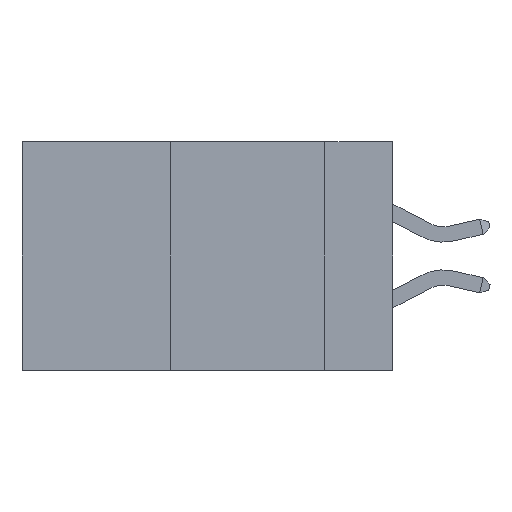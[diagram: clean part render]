
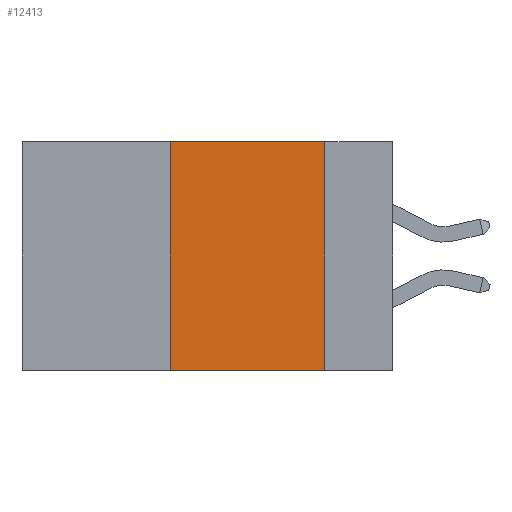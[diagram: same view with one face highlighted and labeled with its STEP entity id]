
A CAD part, left-side view. The second image highlights one B-rep face of the part: STEP entity #12413.
In plain terms, the highlighted planar face has unit normal (-1, 0, 0).
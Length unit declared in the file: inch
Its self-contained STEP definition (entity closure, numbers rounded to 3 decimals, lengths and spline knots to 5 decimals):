
#387 = LINE ( 'NONE', #16037, #11804 ) ;
#531 = EDGE_CURVE ( 'NONE', #13870, #1696, #387, .T. ) ;
#978 = CARTESIAN_POINT ( 'NONE',  ( 0., 0.6, -0.37 ) ) ;
#1008 = CARTESIAN_POINT ( 'NONE',  ( 0., 0.6, 0. ) ) ;
#1041 = EDGE_CURVE ( 'NONE', #1696, #4029, #7498, .T. ) ;
#1696 = VERTEX_POINT ( 'NONE', #3296 ) ;
#2862 = AXIS2_PLACEMENT_3D ( 'NONE', #1008, #8720, #8781 ) ;
#2865 = ORIENTED_EDGE ( 'NONE', *, *, #4188, .T. ) ;
#3212 = VERTEX_POINT ( 'NONE', #8947 ) ;
#3296 = CARTESIAN_POINT ( 'NONE',  ( 0., 0.11, 0. ) ) ;
#4016 = DIRECTION ( 'NONE',  ( 0., -1., 0. ) ) ;
#4029 = VERTEX_POINT ( 'NONE', #18912 ) ;
#4188 = EDGE_CURVE ( 'NONE', #3212, #4029, #18372, .T. ) ;
#6347 = CARTESIAN_POINT ( 'NONE',  ( 0., 0.11, 0. ) ) ;
#6585 = LINE ( 'NONE', #16337, #11335 ) ;
#7106 = FACE_OUTER_BOUND ( 'NONE', #11029, .T. ) ;
#7338 = ORIENTED_EDGE ( 'NONE', *, *, #531, .F. ) ;
#7498 = LINE ( 'NONE', #6347, #13186 ) ;
#8720 = DIRECTION ( 'NONE',  ( 1., 0., 0. ) ) ;
#8781 = DIRECTION ( 'NONE',  ( 0., 0., -1. ) ) ;
#8947 = CARTESIAN_POINT ( 'NONE',  ( 0., 0.36, -0.37 ) ) ;
#9289 = ORIENTED_EDGE ( 'NONE', *, *, #13616, .F. ) ;
#10104 = PLANE ( 'NONE',  #2862 ) ;
#10910 = DIRECTION ( 'NONE',  ( 0., 0., -1. ) ) ;
#11029 = EDGE_LOOP ( 'NONE', ( #13820, #7338, #9289, #2865 ) ) ;
#11335 = VECTOR ( 'NONE', #17888, 39.37008 ) ;
#11804 = VECTOR ( 'NONE', #19195, 39.37008 ) ;
#12413 = ADVANCED_FACE ( 'NONE', ( #7106 ), #10104, .F. ) ;
#13186 = VECTOR ( 'NONE', #10910, 39.37008 ) ;
#13616 = EDGE_CURVE ( 'NONE', #3212, #13870, #6585, .T. ) ;
#13820 = ORIENTED_EDGE ( 'NONE', *, *, #1041, .F. ) ;
#13870 = VERTEX_POINT ( 'NONE', #18229 ) ;
#16037 = CARTESIAN_POINT ( 'NONE',  ( 0., 0.6, 0. ) ) ;
#16337 = CARTESIAN_POINT ( 'NONE',  ( 0., 0.36, 0. ) ) ;
#17888 = DIRECTION ( 'NONE',  ( 0., 0., 1. ) ) ;
#17897 = VECTOR ( 'NONE', #4016, 39.37008 ) ;
#18229 = CARTESIAN_POINT ( 'NONE',  ( 0., 0.36, 0. ) ) ;
#18372 = LINE ( 'NONE', #978, #17897 ) ;
#18912 = CARTESIAN_POINT ( 'NONE',  ( 0., 0.11, -0.37 ) ) ;
#19195 = DIRECTION ( 'NONE',  ( 0., -1., 0. ) ) ;
